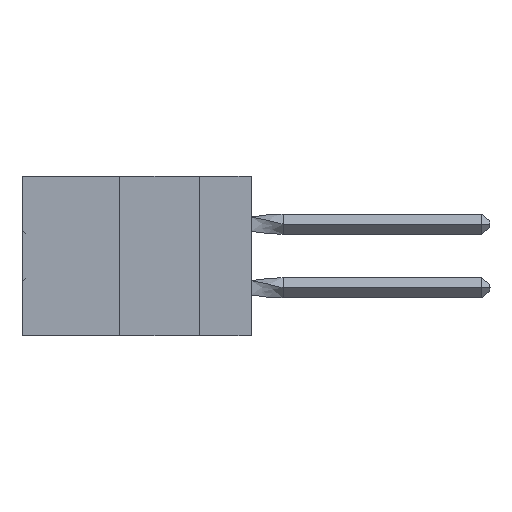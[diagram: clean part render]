
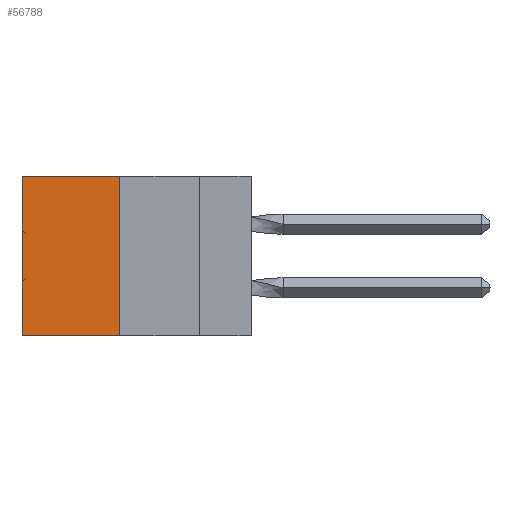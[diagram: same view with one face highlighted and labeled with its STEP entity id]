
A CAD part, left-side view. The second image highlights one B-rep face of the part: STEP entity #56788.
In plain terms, the highlighted planar face has unit normal (-1, 0, 0).
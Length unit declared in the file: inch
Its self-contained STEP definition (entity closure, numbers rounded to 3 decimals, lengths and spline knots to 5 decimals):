
#745 = VECTOR ( 'NONE', #52858, 39.37008 ) ;
#1305 = CARTESIAN_POINT ( 'NONE',  ( 0.305, 0.413, 0. ) ) ;
#2427 = CARTESIAN_POINT ( 'NONE',  ( 0.305, 0.413, 0. ) ) ;
#2499 = AXIS2_PLACEMENT_3D ( 'NONE', #39280, #53611, #24347 ) ;
#2928 = FACE_OUTER_BOUND ( 'NONE', #37104, .T. ) ;
#5554 = DIRECTION ( 'NONE',  ( 0., 0., -1. ) ) ;
#9349 = DIRECTION ( 'NONE',  ( 0., 1., 0. ) ) ;
#10692 = EDGE_CURVE ( 'NONE', #34155, #36500, #46531, .T. ) ;
#10749 = EDGE_CURVE ( 'NONE', #36500, #31888, #12893, .T. ) ;
#12893 = LINE ( 'NONE', #13665, #745 ) ;
#13665 = CARTESIAN_POINT ( 'NONE',  ( 0.305, 0.72, -0.5 ) ) ;
#16597 = DIRECTION ( 'NONE',  ( 0., 1., 0. ) ) ;
#17687 = VECTOR ( 'NONE', #5554, 39.37008 ) ;
#22660 = ORIENTED_EDGE ( 'NONE', *, *, #10749, .T. ) ;
#24347 = DIRECTION ( 'NONE',  ( 0., 0., -1. ) ) ;
#25089 = VECTOR ( 'NONE', #16597, 39.37008 ) ;
#25133 = ORIENTED_EDGE ( 'NONE', *, *, #50143, .F. ) ;
#26579 = CARTESIAN_POINT ( 'NONE',  ( 0.305, 0.72, -0.5 ) ) ;
#27718 = VERTEX_POINT ( 'NONE', #40702 ) ;
#31888 = VERTEX_POINT ( 'NONE', #26579 ) ;
#34155 = VERTEX_POINT ( 'NONE', #2427 ) ;
#36500 = VERTEX_POINT ( 'NONE', #58943 ) ;
#37104 = EDGE_LOOP ( 'NONE', ( #22660, #62246, #25133, #40897 ) ) ;
#39280 = CARTESIAN_POINT ( 'NONE',  ( 0.305, 0.413, -0.5 ) ) ;
#39617 = EDGE_CURVE ( 'NONE', #27718, #31888, #43175, .T. ) ;
#40271 = CARTESIAN_POINT ( 'NONE',  ( 0.305, 0.413, -0.5 ) ) ;
#40596 = LINE ( 'NONE', #40271, #17687 ) ;
#40702 = CARTESIAN_POINT ( 'NONE',  ( 0.305, 0.413, -0.5 ) ) ;
#40897 = ORIENTED_EDGE ( 'NONE', *, *, #10692, .T. ) ;
#43175 = LINE ( 'NONE', #53434, #54630 ) ;
#46531 = LINE ( 'NONE', #1305, #25089 ) ;
#50143 = EDGE_CURVE ( 'NONE', #34155, #27718, #40596, .T. ) ;
#52858 = DIRECTION ( 'NONE',  ( 0., 0., -1. ) ) ;
#53434 = CARTESIAN_POINT ( 'NONE',  ( 0.305, 0.413, -0.5 ) ) ;
#53611 = DIRECTION ( 'NONE',  ( 1., 0., 0. ) ) ;
#54630 = VECTOR ( 'NONE', #9349, 39.37008 ) ;
#56788 = ADVANCED_FACE ( 'NONE', ( #2928 ), #58321, .F. ) ;
#58321 = PLANE ( 'NONE',  #2499 ) ;
#58943 = CARTESIAN_POINT ( 'NONE',  ( 0.305, 0.72, 0. ) ) ;
#62246 = ORIENTED_EDGE ( 'NONE', *, *, #39617, .F. ) ;
